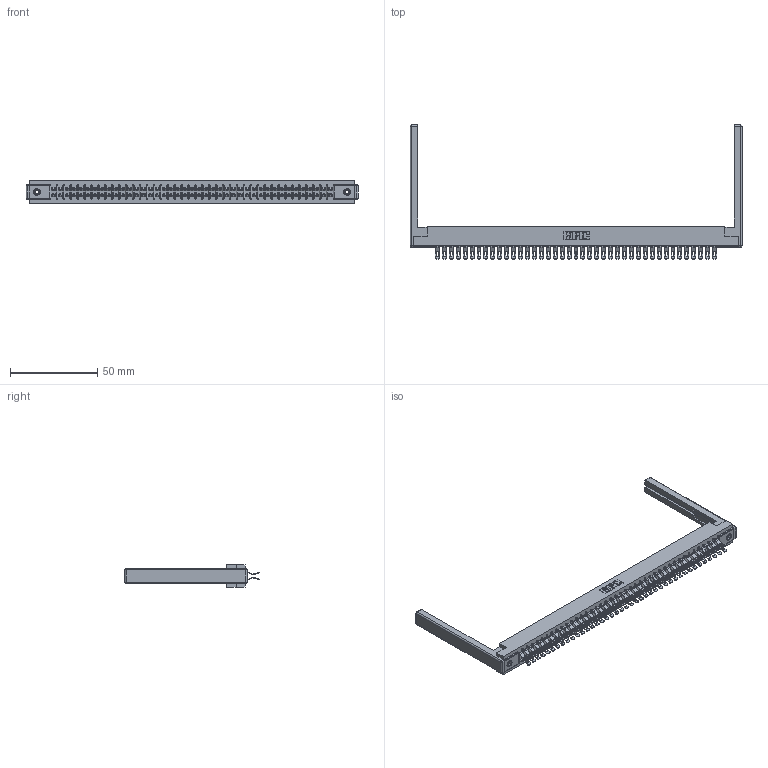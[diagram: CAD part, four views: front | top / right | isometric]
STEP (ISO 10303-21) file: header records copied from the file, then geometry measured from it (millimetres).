
FILE_DESCRIPTION (( 'STEP AP203' ), '1' );
FILE_NAME ('357-082-555-268.STEP', '2019-09-19T17:00:22', ( '' ), ( '' ), 'SwSTEP 2.0', 'SolidWorks 2016', '' );
FILE_SCHEMA (( 'CONFIG_CONTROL_DESIGN' ));
Length unit declared in the file: inch
Products named in the file (5): 307-220-068; 357-082-555-268; 307-290-001_555; 345-250-001_345-250-001-102; 307 Part_.156 Dia Mounting Holes
Assembly tree (87 placements, depth 2):
  357-082-555-268
    307 Part_.156 Dia Mounting Holes
    307-290-001_555  x82
    307-220-068  x2
    345-250-001_345-250-001-102  x2
Bounding box: 189.89 x 76.71 x 12.7 mm (x, y, z)
Volume: 24810.4 mm3; surface area: 30314.8 mm2
Topology: 87 solids, 87 shells, 5316 faces, 15555 edges, 10126 vertices
Faces by surface type: plane 2946, cylinder 2262, sphere 92, cone 12, torus 4
Entity records: 39880 total; most frequent: CARTESIAN_POINT 6506, ORIENTED_EDGE 6442, DIRECTION 6395, EDGE_CURVE 3221, LINE 2457, VECTOR 2457, VERTEX_POINT 2080, AXIS2_PLACEMENT_3D 1969
